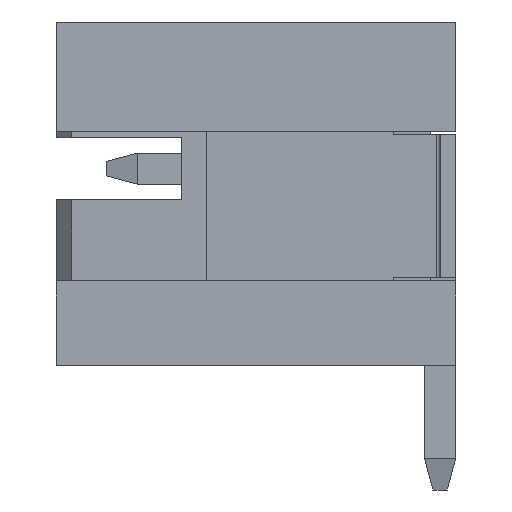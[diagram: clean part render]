
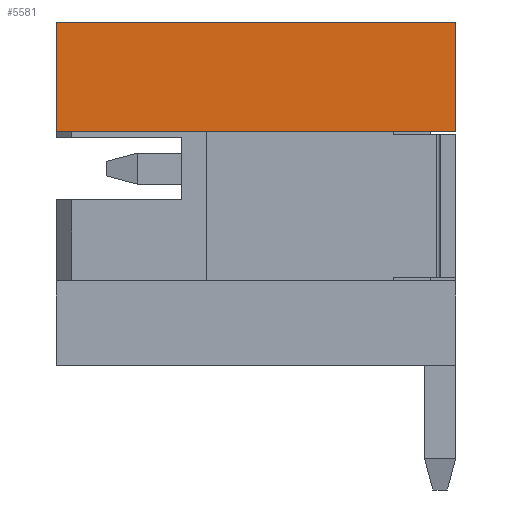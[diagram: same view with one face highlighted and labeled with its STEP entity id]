
A CAD part, left-side view. The second image highlights one B-rep face of the part: STEP entity #5581.
In plain terms, the highlighted planar face has unit normal (-1, 0, 0).
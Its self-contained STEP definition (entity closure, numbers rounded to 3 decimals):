
#89 = PLANE ( 'NONE',  #3937 ) ;
#931 = VERTEX_POINT ( 'NONE', #1903 ) ;
#961 = DIRECTION ( 'NONE',  ( 0., -1., 0. ) ) ;
#992 = LINE ( 'NONE', #3142, #3398 ) ;
#1003 = EDGE_CURVE ( 'NONE', #2191, #1662, #3664, .T. ) ;
#1078 = FACE_OUTER_BOUND ( 'NONE', #5211, .T. ) ;
#1135 = DIRECTION ( 'NONE',  ( 1., 0., 0. ) ) ;
#1412 = ORIENTED_EDGE ( 'NONE', *, *, #5686, .F. ) ;
#1611 = LINE ( 'NONE', #3694, #5165 ) ;
#1662 = VERTEX_POINT ( 'NONE', #4393 ) ;
#1903 = CARTESIAN_POINT ( 'NONE',  ( -3., 0., 2.35 ) ) ;
#2191 = VERTEX_POINT ( 'NONE', #4805 ) ;
#2215 = ORIENTED_EDGE ( 'NONE', *, *, #2275, .F. ) ;
#2275 = EDGE_CURVE ( 'NONE', #1662, #931, #1611, .T. ) ;
#2429 = DIRECTION ( 'NONE',  ( 0., 0., 1. ) ) ;
#2527 = CARTESIAN_POINT ( 'NONE',  ( -3., 0., 0.6 ) ) ;
#2820 = VERTEX_POINT ( 'NONE', #5241 ) ;
#2910 = ORIENTED_EDGE ( 'NONE', *, *, #3907, .F. ) ;
#3142 = CARTESIAN_POINT ( 'NONE',  ( -3., 0., 2.35 ) ) ;
#3398 = VECTOR ( 'NONE', #5071, 1000. ) ;
#3455 = DIRECTION ( 'NONE',  ( 0., 1., 0. ) ) ;
#3639 = ORIENTED_EDGE ( 'NONE', *, *, #1003, .F. ) ;
#3664 = LINE ( 'NONE', #5196, #5901 ) ;
#3683 = VECTOR ( 'NONE', #3455, 1000. ) ;
#3694 = CARTESIAN_POINT ( 'NONE',  ( -3., 6.4, 2.35 ) ) ;
#3907 = EDGE_CURVE ( 'NONE', #931, #2820, #992, .T. ) ;
#3922 = CARTESIAN_POINT ( 'NONE',  ( -3., 0., 0. ) ) ;
#3937 = AXIS2_PLACEMENT_3D ( 'NONE', #3922, #1135, #5710 ) ;
#4393 = CARTESIAN_POINT ( 'NONE',  ( -3., 6.4, 2.35 ) ) ;
#4805 = CARTESIAN_POINT ( 'NONE',  ( -3., 6.4, 0.6 ) ) ;
#5071 = DIRECTION ( 'NONE',  ( 0., 0., -1. ) ) ;
#5165 = VECTOR ( 'NONE', #961, 1000. ) ;
#5196 = CARTESIAN_POINT ( 'NONE',  ( -3., 6.4, 2.35 ) ) ;
#5203 = LINE ( 'NONE', #2527, #3683 ) ;
#5211 = EDGE_LOOP ( 'NONE', ( #3639, #1412, #2910, #2215 ) ) ;
#5241 = CARTESIAN_POINT ( 'NONE',  ( -3., 0., 0.6 ) ) ;
#5581 = ADVANCED_FACE ( 'NONE', ( #1078 ), #89, .F. ) ;
#5686 = EDGE_CURVE ( 'NONE', #2820, #2191, #5203, .T. ) ;
#5710 = DIRECTION ( 'NONE',  ( 0., 0., -1. ) ) ;
#5901 = VECTOR ( 'NONE', #2429, 1000. ) ;
